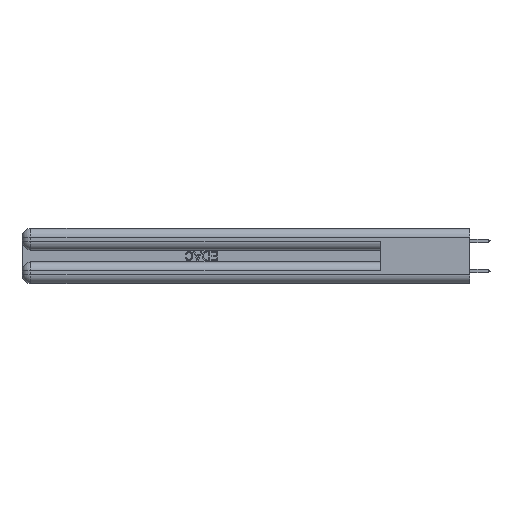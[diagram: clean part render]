
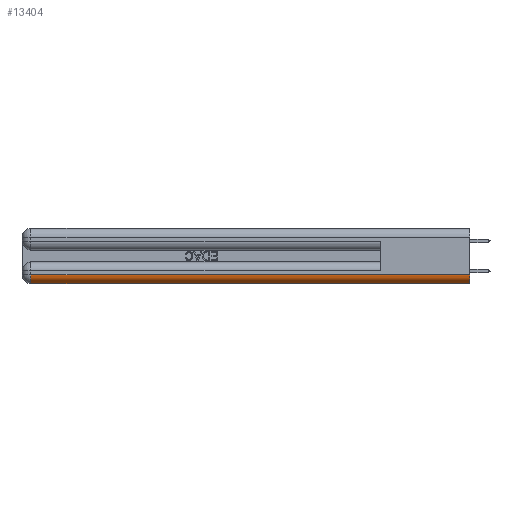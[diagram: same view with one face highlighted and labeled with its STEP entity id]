
A CAD part, left-side view. The second image highlights one B-rep face of the part: STEP entity #13404.
In plain terms, the highlighted cylindrical face has radius 1.524 mm (diameter 3.048 mm), a partial arc.
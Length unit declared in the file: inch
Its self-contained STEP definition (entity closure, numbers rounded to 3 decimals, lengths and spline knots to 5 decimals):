
#634 = EDGE_LOOP ( 'NONE', ( #24145, #33747, #32042, #26062 ) ) ;
#1703 = CIRCLE ( 'NONE', #13097, 0.06 ) ;
#1745 = EDGE_CURVE ( 'NONE', #4700, #19693, #1703, .T. ) ;
#2573 = DIRECTION ( 'NONE',  ( 0., 0., 1. ) ) ;
#4700 = VERTEX_POINT ( 'NONE', #25481 ) ;
#6005 = DIRECTION ( 'NONE',  ( 0., -1., 0. ) ) ;
#6647 = DIRECTION ( 'NONE',  ( 0., 0., 1. ) ) ;
#7514 = FACE_OUTER_BOUND ( 'NONE', #634, .T. ) ;
#7633 = VERTEX_POINT ( 'NONE', #36243 ) ;
#9065 = LINE ( 'NONE', #40858, #25093 ) ;
#11038 = CARTESIAN_POINT ( 'NONE',  ( 0.06, 0., 0.06 ) ) ;
#11239 = CYLINDRICAL_SURFACE ( 'NONE', #36724, 0.06 ) ;
#11981 = CARTESIAN_POINT ( 'NONE',  ( 0., 0., 0.06 ) ) ;
#13097 = AXIS2_PLACEMENT_3D ( 'NONE', #30761, #43911, #6647 ) ;
#13189 = EDGE_CURVE ( 'NONE', #7633, #4700, #9065, .T. ) ;
#13404 = ADVANCED_FACE ( 'NONE', ( #7514 ), #11239, .T. ) ;
#17909 = VECTOR ( 'NONE', #41286, 39.37008 ) ;
#19693 = VERTEX_POINT ( 'NONE', #42376 ) ;
#19727 = AXIS2_PLACEMENT_3D ( 'NONE', #30127, #6005, #2573 ) ;
#23326 = LINE ( 'NONE', #24882, #17909 ) ;
#24145 = ORIENTED_EDGE ( 'NONE', *, *, #32487, .F. ) ;
#24882 = CARTESIAN_POINT ( 'NONE',  ( 0., 0., 0.06 ) ) ;
#25093 = VECTOR ( 'NONE', #37597, 39.37008 ) ;
#25481 = CARTESIAN_POINT ( 'NONE',  ( 0.06, 2.94, 0. ) ) ;
#25520 = VERTEX_POINT ( 'NONE', #11981 ) ;
#26062 = ORIENTED_EDGE ( 'NONE', *, *, #13189, .F. ) ;
#30127 = CARTESIAN_POINT ( 'NONE',  ( 0.06, 0., 0.06 ) ) ;
#30761 = CARTESIAN_POINT ( 'NONE',  ( 0.06, 2.94, 0.06 ) ) ;
#32042 = ORIENTED_EDGE ( 'NONE', *, *, #1745, .F. ) ;
#32487 = EDGE_CURVE ( 'NONE', #25520, #7633, #38069, .T. ) ;
#32547 = DIRECTION ( 'NONE',  ( 0., 0., 1. ) ) ;
#33747 = ORIENTED_EDGE ( 'NONE', *, *, #37709, .F. ) ;
#36243 = CARTESIAN_POINT ( 'NONE',  ( 0.06, 0., 0. ) ) ;
#36724 = AXIS2_PLACEMENT_3D ( 'NONE', #11038, #41877, #32547 ) ;
#37597 = DIRECTION ( 'NONE',  ( 0., 1., 0. ) ) ;
#37709 = EDGE_CURVE ( 'NONE', #19693, #25520, #23326, .T. ) ;
#38069 = CIRCLE ( 'NONE', #19727, 0.06 ) ;
#40858 = CARTESIAN_POINT ( 'NONE',  ( 0.06, 3., 0. ) ) ;
#41286 = DIRECTION ( 'NONE',  ( 0., -1., 0. ) ) ;
#41877 = DIRECTION ( 'NONE',  ( 0., 1., 0. ) ) ;
#42376 = CARTESIAN_POINT ( 'NONE',  ( 0., 2.94, 0.06 ) ) ;
#43911 = DIRECTION ( 'NONE',  ( 0., 1., 0. ) ) ;
